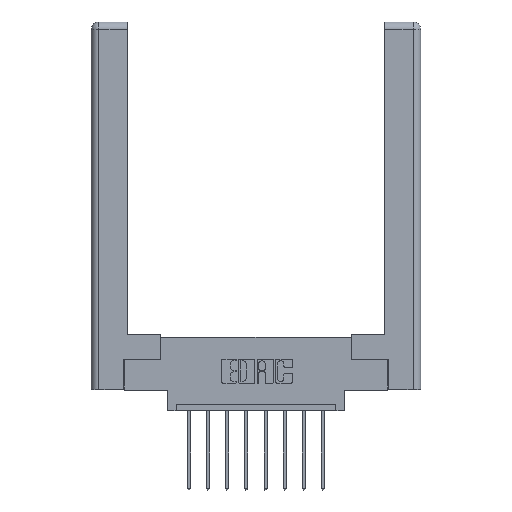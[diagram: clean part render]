
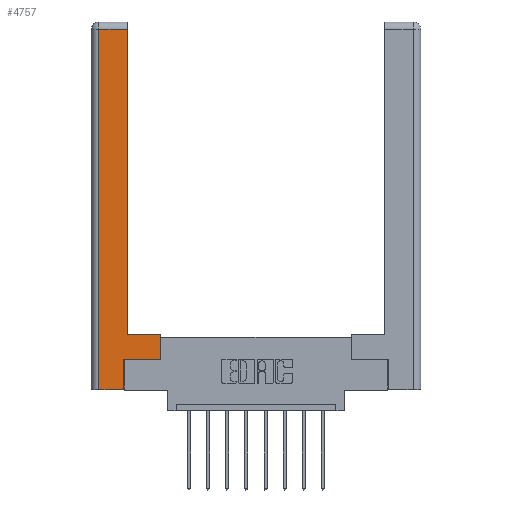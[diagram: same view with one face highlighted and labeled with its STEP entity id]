
A CAD part, top view. The second image highlights one B-rep face of the part: STEP entity #4757.
In plain terms, the highlighted planar face has unit normal (0, 0, 1).
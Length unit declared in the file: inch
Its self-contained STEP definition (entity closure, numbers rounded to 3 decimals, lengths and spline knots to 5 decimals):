
#128 = ORIENTED_EDGE ( 'NONE', *, *, #5425, .T. ) ;
#150 = EDGE_CURVE ( 'NONE', #1488, #11936, #278, .T. ) ;
#278 = LINE ( 'NONE', #6137, #3593 ) ;
#304 = EDGE_CURVE ( 'NONE', #4150, #3863, #900, .T. ) ;
#819 = ORIENTED_EDGE ( 'NONE', *, *, #9188, .T. ) ;
#900 = LINE ( 'NONE', #7036, #10442 ) ;
#921 = LINE ( 'NONE', #5846, #10465 ) ;
#1204 = VECTOR ( 'NONE', #12416, 39.37008 ) ;
#1488 = VERTEX_POINT ( 'NONE', #3685 ) ;
#1676 = EDGE_CURVE ( 'NONE', #10259, #5413, #9501, .T. ) ;
#1828 = CARTESIAN_POINT ( 'NONE',  ( 0.295, 2.94, 0. ) ) ;
#2655 = VECTOR ( 'NONE', #2675, 39.37008 ) ;
#2675 = DIRECTION ( 'NONE',  ( -1., 0., 0. ) ) ;
#3038 = DIRECTION ( 'NONE',  ( 0., 1., 0. ) ) ;
#3109 = ORIENTED_EDGE ( 'NONE', *, *, #3122, .T. ) ;
#3122 = EDGE_CURVE ( 'NONE', #3863, #7215, #4535, .T. ) ;
#3593 = VECTOR ( 'NONE', #7149, 39.37008 ) ;
#3685 = CARTESIAN_POINT ( 'NONE',  ( 0.295, 0.45, 0. ) ) ;
#3710 = ORIENTED_EDGE ( 'NONE', *, *, #10731, .T. ) ;
#3863 = VERTEX_POINT ( 'NONE', #7063 ) ;
#4051 = CARTESIAN_POINT ( 'NONE',  ( 0.565, 0.45, 0. ) ) ;
#4150 = VERTEX_POINT ( 'NONE', #9379 ) ;
#4333 = PLANE ( 'NONE',  #5714 ) ;
#4535 = LINE ( 'NONE', #4647, #7378 ) ;
#4647 = CARTESIAN_POINT ( 'NONE',  ( 0.265, 0., 0. ) ) ;
#4757 = ADVANCED_FACE ( 'NONE', ( #7996 ), #4333, .F. ) ;
#4780 = DIRECTION ( 'NONE',  ( -1., 0., 0. ) ) ;
#5334 = VECTOR ( 'NONE', #7372, 39.37008 ) ;
#5355 = CARTESIAN_POINT ( 'NONE',  ( 0., 0., 0. ) ) ;
#5413 = VERTEX_POINT ( 'NONE', #4051 ) ;
#5425 = EDGE_CURVE ( 'NONE', #7215, #10851, #12715, .T. ) ;
#5665 = LINE ( 'NONE', #9562, #1204 ) ;
#5714 = AXIS2_PLACEMENT_3D ( 'NONE', #5355, #6341, #10387 ) ;
#5846 = CARTESIAN_POINT ( 'NONE',  ( 0.295, 0.45, 0. ) ) ;
#5995 = ORIENTED_EDGE ( 'NONE', *, *, #1676, .T. ) ;
#6137 = CARTESIAN_POINT ( 'NONE',  ( 0.295, 3., 0. ) ) ;
#6341 = DIRECTION ( 'NONE',  ( 0., 0., -1. ) ) ;
#7036 = CARTESIAN_POINT ( 'NONE',  ( 0.0615, 0., 0. ) ) ;
#7063 = CARTESIAN_POINT ( 'NONE',  ( 0.0615, 0., 0. ) ) ;
#7149 = DIRECTION ( 'NONE',  ( 0., 1., 0. ) ) ;
#7215 = VERTEX_POINT ( 'NONE', #7819 ) ;
#7274 = LINE ( 'NONE', #7770, #2655 ) ;
#7327 = CARTESIAN_POINT ( 'NONE',  ( 0.565, 0.45, 0. ) ) ;
#7372 = DIRECTION ( 'NONE',  ( 0., 1., 0. ) ) ;
#7378 = VECTOR ( 'NONE', #8613, 39.37008 ) ;
#7770 = CARTESIAN_POINT ( 'NONE',  ( 0.0615, 2.94, 0. ) ) ;
#7819 = CARTESIAN_POINT ( 'NONE',  ( 0.265, 0., 0. ) ) ;
#7823 = VECTOR ( 'NONE', #3038, 39.37008 ) ;
#7996 = FACE_OUTER_BOUND ( 'NONE', #10549, .T. ) ;
#8613 = DIRECTION ( 'NONE',  ( 1., 0., 0. ) ) ;
#8619 = ORIENTED_EDGE ( 'NONE', *, *, #150, .T. ) ;
#9188 = EDGE_CURVE ( 'NONE', #11936, #4150, #7274, .T. ) ;
#9266 = EDGE_CURVE ( 'NONE', #5413, #1488, #921, .T. ) ;
#9379 = CARTESIAN_POINT ( 'NONE',  ( 0.0615, 2.94, 0. ) ) ;
#9501 = LINE ( 'NONE', #7327, #5334 ) ;
#9562 = CARTESIAN_POINT ( 'NONE',  ( 0.565, 0.245, 0. ) ) ;
#10259 = VERTEX_POINT ( 'NONE', #11732 ) ;
#10387 = DIRECTION ( 'NONE',  ( -1., 0., 0. ) ) ;
#10442 = VECTOR ( 'NONE', #12480, 39.37008 ) ;
#10465 = VECTOR ( 'NONE', #4780, 39.37008 ) ;
#10549 = EDGE_LOOP ( 'NONE', ( #8619, #819, #11829, #3109, #128, #3710, #5995, #11649 ) ) ;
#10731 = EDGE_CURVE ( 'NONE', #10851, #10259, #5665, .T. ) ;
#10851 = VERTEX_POINT ( 'NONE', #11718 ) ;
#11151 = CARTESIAN_POINT ( 'NONE',  ( 0.265, 0.245, 0. ) ) ;
#11649 = ORIENTED_EDGE ( 'NONE', *, *, #9266, .T. ) ;
#11718 = CARTESIAN_POINT ( 'NONE',  ( 0.265, 0.245, 0. ) ) ;
#11732 = CARTESIAN_POINT ( 'NONE',  ( 0.565, 0.245, 0. ) ) ;
#11829 = ORIENTED_EDGE ( 'NONE', *, *, #304, .T. ) ;
#11936 = VERTEX_POINT ( 'NONE', #1828 ) ;
#12416 = DIRECTION ( 'NONE',  ( 1., 0., 0. ) ) ;
#12480 = DIRECTION ( 'NONE',  ( 0., -1., 0. ) ) ;
#12715 = LINE ( 'NONE', #11151, #7823 ) ;
